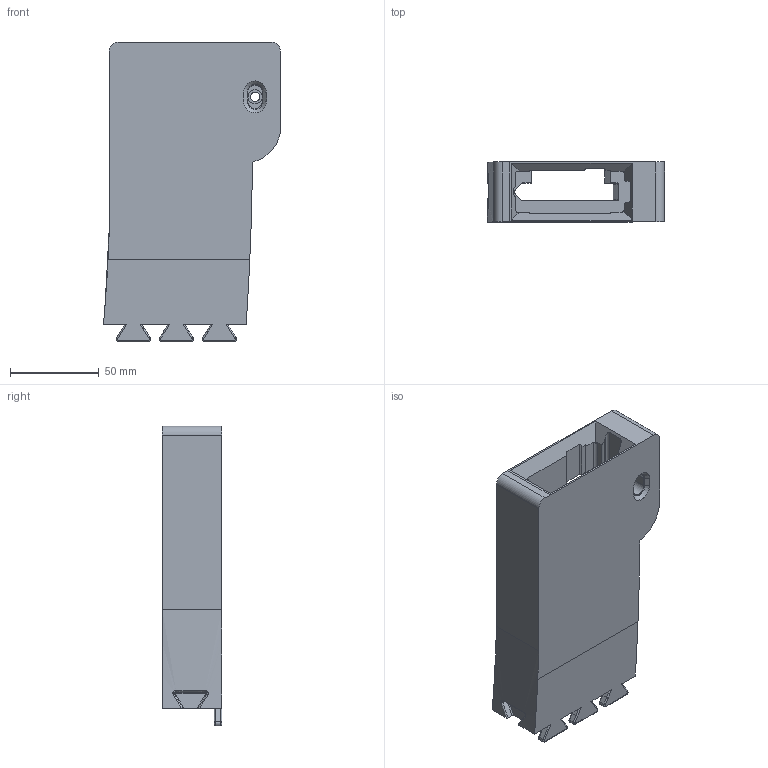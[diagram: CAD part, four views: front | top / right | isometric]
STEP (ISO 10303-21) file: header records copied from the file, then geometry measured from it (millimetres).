
FILE_DESCRIPTION(/* description */ (''),/* implementation_level */ '2;1');
FILE_NAME(/* name */ 'freeman1337_ar15-mag-speedloader-base-engraved-v5.step',/* time_stamp */ '2021-09-04T08:15:36-07:00',/* author */ (''),/* organization */ (''),/* preprocessor_version */ 'ST-DEVELOPER v18.1',/* originating_system */ 'Autodesk Translation Framework v10.10.0.1391',/* authorisation */ '');
FILE_SCHEMA (('AUTOMOTIVE_DESIGN { 1 0 10303 214 3 1 1 }'));
Products named in the file (1): loader-base-engraved
Bounding box: 99.63 x 33.62 x 168.54 mm (x, y, z)
Volume: 254302.8 mm3; surface area: 62970.9 mm2
Topology: 1 solids, 2 shells, 3314 faces, 9092 edges, 6034 vertices
Faces by surface type: bspline 2379, plane 840, cylinder 87, cone 6, torus 1, sphere 1
Full cylindrical faces by diameter (mm): 5.182 x1, 7.925 x1
Entity records: 113779 total; most frequent: CARTESIAN_POINT 50565, ORIENTED_EDGE 18184, EDGE_CURVE 9092, DIRECTION 7079, VERTEX_POINT 6034, LINE 4161, VECTOR 4161, EDGE_LOOP 3572
